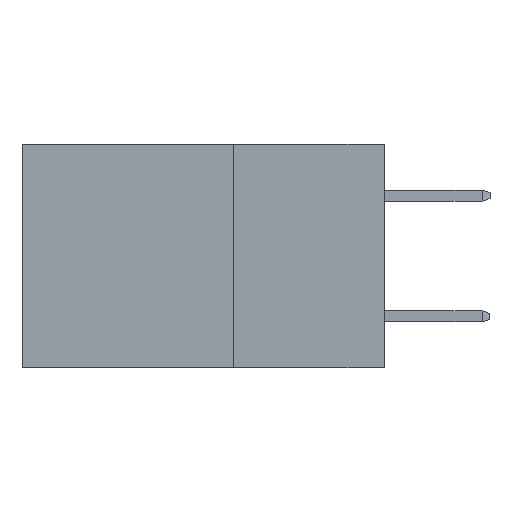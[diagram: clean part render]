
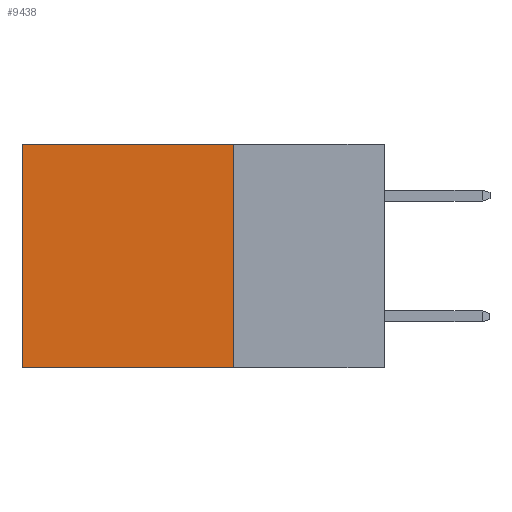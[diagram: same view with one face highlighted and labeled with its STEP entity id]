
A CAD part, left-side view. The second image highlights one B-rep face of the part: STEP entity #9438.
In plain terms, the highlighted planar face has unit normal (-1, 0, 0).
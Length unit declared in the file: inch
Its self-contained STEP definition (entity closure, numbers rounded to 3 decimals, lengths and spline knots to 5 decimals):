
#434 = VECTOR ( 'NONE', #3185, 39.37008 ) ;
#793 = FACE_OUTER_BOUND ( 'NONE', #1040, .T. ) ;
#1040 = EDGE_LOOP ( 'NONE', ( #6789, #6590, #8072, #11308 ) ) ;
#1927 = DIRECTION ( 'NONE',  ( 0., 0., -1. ) ) ;
#2025 = DIRECTION ( 'NONE',  ( 0., 0., -1. ) ) ;
#2303 = LINE ( 'NONE', #13001, #4122 ) ;
#2306 = CARTESIAN_POINT ( 'NONE',  ( 0.298, 0.6, 0. ) ) ;
#2419 = VERTEX_POINT ( 'NONE', #7517 ) ;
#2839 = CARTESIAN_POINT ( 'NONE',  ( 0.298, 0.25, -0.37 ) ) ;
#3092 = EDGE_CURVE ( 'NONE', #6053, #3237, #2303, .T. ) ;
#3185 = DIRECTION ( 'NONE',  ( 0., 0., -1. ) ) ;
#3237 = VERTEX_POINT ( 'NONE', #2306 ) ;
#4122 = VECTOR ( 'NONE', #12870, 39.37008 ) ;
#5283 = EDGE_CURVE ( 'NONE', #6053, #9942, #9416, .T. ) ;
#6053 = VERTEX_POINT ( 'NONE', #9354 ) ;
#6063 = LINE ( 'NONE', #8338, #434 ) ;
#6590 = ORIENTED_EDGE ( 'NONE', *, *, #11272, .F. ) ;
#6789 = ORIENTED_EDGE ( 'NONE', *, *, #12022, .T. ) ;
#6893 = VECTOR ( 'NONE', #12859, 39.37008 ) ;
#7163 = CARTESIAN_POINT ( 'NONE',  ( 0.298, 0.25, 0. ) ) ;
#7517 = CARTESIAN_POINT ( 'NONE',  ( 0.298, 0.6, -0.37 ) ) ;
#8072 = ORIENTED_EDGE ( 'NONE', *, *, #5283, .F. ) ;
#8182 = DIRECTION ( 'NONE',  ( 1., 0., 0. ) ) ;
#8338 = CARTESIAN_POINT ( 'NONE',  ( 0.298, 0.6, 0. ) ) ;
#9222 = AXIS2_PLACEMENT_3D ( 'NONE', #7163, #8182, #1927 ) ;
#9354 = CARTESIAN_POINT ( 'NONE',  ( 0.298, 0.25, 0. ) ) ;
#9416 = LINE ( 'NONE', #11121, #11650 ) ;
#9438 = ADVANCED_FACE ( 'NONE', ( #793 ), #12988, .F. ) ;
#9465 = LINE ( 'NONE', #2839, #6893 ) ;
#9942 = VERTEX_POINT ( 'NONE', #11719 ) ;
#11121 = CARTESIAN_POINT ( 'NONE',  ( 0.298, 0.25, 0. ) ) ;
#11272 = EDGE_CURVE ( 'NONE', #9942, #2419, #9465, .T. ) ;
#11308 = ORIENTED_EDGE ( 'NONE', *, *, #3092, .T. ) ;
#11650 = VECTOR ( 'NONE', #2025, 39.37008 ) ;
#11719 = CARTESIAN_POINT ( 'NONE',  ( 0.298, 0.25, -0.37 ) ) ;
#12022 = EDGE_CURVE ( 'NONE', #3237, #2419, #6063, .T. ) ;
#12859 = DIRECTION ( 'NONE',  ( 0., 1., 0. ) ) ;
#12870 = DIRECTION ( 'NONE',  ( 0., 1., 0. ) ) ;
#12988 = PLANE ( 'NONE',  #9222 ) ;
#13001 = CARTESIAN_POINT ( 'NONE',  ( 0.298, 0.25, 0. ) ) ;
